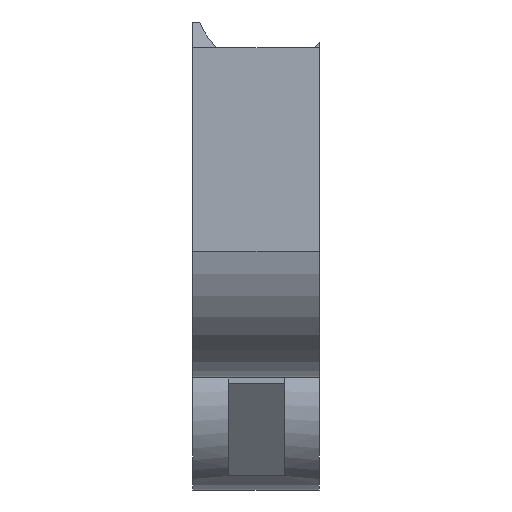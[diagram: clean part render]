
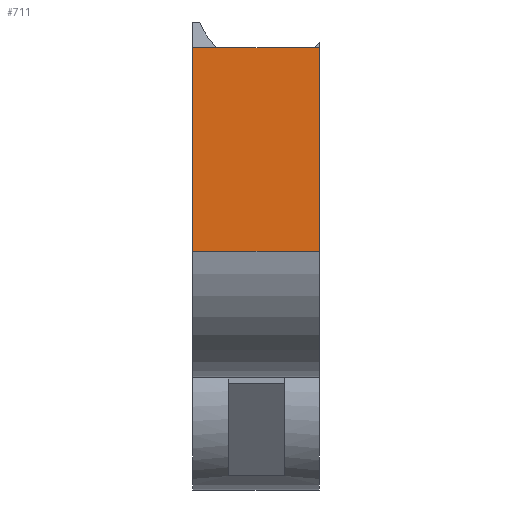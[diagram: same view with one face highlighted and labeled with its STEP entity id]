
A CAD part, left-side view. The second image highlights one B-rep face of the part: STEP entity #711.
In plain terms, the highlighted planar face has unit normal (-1, 0, 0).
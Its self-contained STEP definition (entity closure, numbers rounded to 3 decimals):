
#10 = ORIENTED_EDGE ( 'NONE', *, *, #264, .T. ) ;
#47 = CARTESIAN_POINT ( 'NONE',  ( -142.125, 29.15, -5.93 ) ) ;
#59 = CARTESIAN_POINT ( 'NONE',  ( -142.125, 28.1, -25.1 ) ) ;
#65 = VERTEX_POINT ( 'NONE', #1344 ) ;
#77 = LINE ( 'NONE', #699, #781 ) ;
#85 = EDGE_LOOP ( 'NONE', ( #1022, #96, #10, #917 ) ) ;
#96 = ORIENTED_EDGE ( 'NONE', *, *, #1168, .T. ) ;
#129 = DIRECTION ( 'NONE',  ( 0., 0., 1. ) ) ;
#238 = VERTEX_POINT ( 'NONE', #287 ) ;
#264 = EDGE_CURVE ( 'NONE', #1249, #665, #77, .T. ) ;
#280 = LINE ( 'NONE', #1092, #1349 ) ;
#287 = CARTESIAN_POINT ( 'NONE',  ( -142.125, 20.1, -20.44 ) ) ;
#300 = VECTOR ( 'NONE', #129, 1000. ) ;
#311 = AXIS2_PLACEMENT_3D ( 'NONE', #59, #602, #803 ) ;
#375 = VECTOR ( 'NONE', #649, 1000. ) ;
#385 = PLANE ( 'NONE',  #311 ) ;
#416 = LINE ( 'NONE', #1270, #375 ) ;
#602 = DIRECTION ( 'NONE',  ( 1., 0., 0. ) ) ;
#649 = DIRECTION ( 'NONE',  ( 0., 1., 0. ) ) ;
#665 = VERTEX_POINT ( 'NONE', #47 ) ;
#699 = CARTESIAN_POINT ( 'NONE',  ( -142.125, 28.1, -5.93 ) ) ;
#711 = ADVANCED_FACE ( 'NONE', ( #1110 ), #385, .F. ) ;
#756 = CARTESIAN_POINT ( 'NONE',  ( -142.125, 20.1, -29.669 ) ) ;
#781 = VECTOR ( 'NONE', #1122, 1000. ) ;
#803 = DIRECTION ( 'NONE',  ( 0., 0., 1. ) ) ;
#880 = LINE ( 'NONE', #756, #300 ) ;
#917 = ORIENTED_EDGE ( 'NONE', *, *, #1015, .F. ) ;
#976 = EDGE_CURVE ( 'NONE', #238, #65, #416, .T. ) ;
#983 = CARTESIAN_POINT ( 'NONE',  ( -142.125, 20.1, -5.93 ) ) ;
#1015 = EDGE_CURVE ( 'NONE', #65, #665, #280, .T. ) ;
#1022 = ORIENTED_EDGE ( 'NONE', *, *, #976, .F. ) ;
#1092 = CARTESIAN_POINT ( 'NONE',  ( -142.125, 29.15, -12.459 ) ) ;
#1110 = FACE_OUTER_BOUND ( 'NONE', #85, .T. ) ;
#1122 = DIRECTION ( 'NONE',  ( 0., 1., 0. ) ) ;
#1168 = EDGE_CURVE ( 'NONE', #238, #1249, #880, .T. ) ;
#1198 = DIRECTION ( 'NONE',  ( 0., 0., 1. ) ) ;
#1249 = VERTEX_POINT ( 'NONE', #983 ) ;
#1270 = CARTESIAN_POINT ( 'NONE',  ( -142.125, 29.15, -20.44 ) ) ;
#1344 = CARTESIAN_POINT ( 'NONE',  ( -142.125, 29.15, -20.44 ) ) ;
#1349 = VECTOR ( 'NONE', #1198, 1000. ) ;
